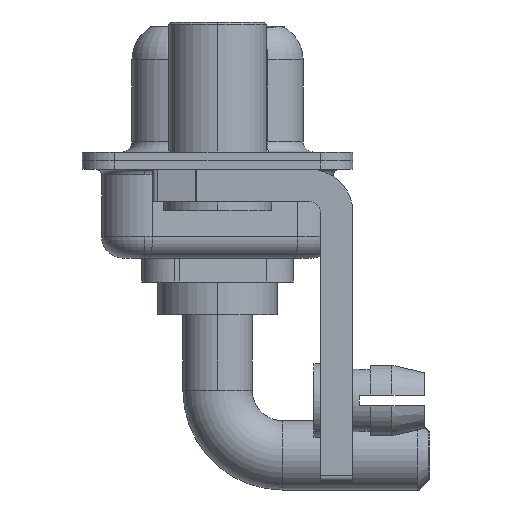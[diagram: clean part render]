
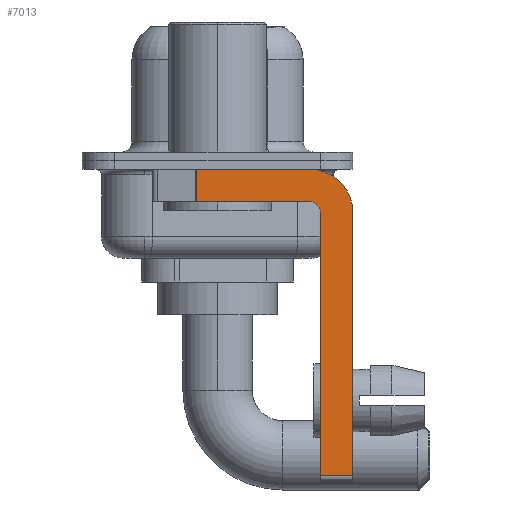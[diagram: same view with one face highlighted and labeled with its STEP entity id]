
A CAD part, left-side view. The second image highlights one B-rep face of the part: STEP entity #7013.
In plain terms, the highlighted planar face has unit normal (-1, 0, 0).
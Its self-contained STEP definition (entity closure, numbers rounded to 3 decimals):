
#165 = AXIS2_PLACEMENT_3D ( 'NONE', #1586, #16486, #4479 ) ;
#211 = CARTESIAN_POINT ( 'NONE',  ( -2.9, -4.25, -2.4 ) ) ;
#673 = LINE ( 'NONE', #15731, #5815 ) ;
#1586 = CARTESIAN_POINT ( 'NONE',  ( -2.9, -4.25, -2.4 ) ) ;
#2033 = CARTESIAN_POINT ( 'NONE',  ( -2.9, -6.25, -2.4 ) ) ;
#2259 = VECTOR ( 'NONE', #5980, 1000. ) ;
#2355 = DIRECTION ( 'NONE',  ( 0., 1., 0. ) ) ;
#2652 = CARTESIAN_POINT ( 'NONE',  ( -2.9, -4.25, -1.9 ) ) ;
#3061 = DIRECTION ( 'NONE',  ( 0., 0., -1. ) ) ;
#3153 = DIRECTION ( 'NONE',  ( 1., 0., 0. ) ) ;
#3361 = LINE ( 'NONE', #2033, #14634 ) ;
#3612 = CARTESIAN_POINT ( 'NONE',  ( -2.9, 0.978, -1.9 ) ) ;
#3843 = ORIENTED_EDGE ( 'NONE', *, *, #8644, .T. ) ;
#4019 = CARTESIAN_POINT ( 'NONE',  ( -2.9, -4.25, -14.55 ) ) ;
#4239 = VECTOR ( 'NONE', #2355, 1000. ) ;
#4290 = CIRCLE ( 'NONE', #7648, 2. ) ;
#4424 = EDGE_CURVE ( 'NONE', #13853, #8016, #9050, .T. ) ;
#4479 = DIRECTION ( 'NONE',  ( 0., 0., 1. ) ) ;
#4519 = AXIS2_PLACEMENT_3D ( 'NONE', #211, #13544, #13622 ) ;
#4754 = ORIENTED_EDGE ( 'NONE', *, *, #17302, .F. ) ;
#4914 = VERTEX_POINT ( 'NONE', #8689 ) ;
#5020 = VECTOR ( 'NONE', #10282, 1000. ) ;
#5219 = ORIENTED_EDGE ( 'NONE', *, *, #14385, .F. ) ;
#5685 = CARTESIAN_POINT ( 'NONE',  ( -2.9, -4.25, -2.4 ) ) ;
#5815 = VECTOR ( 'NONE', #13022, 1000. ) ;
#5980 = DIRECTION ( 'NONE',  ( 0., 0., 1. ) ) ;
#6066 = ORIENTED_EDGE ( 'NONE', *, *, #10455, .F. ) ;
#6239 = CARTESIAN_POINT ( 'NONE',  ( -2.9, -4.75, -14.8 ) ) ;
#6323 = VERTEX_POINT ( 'NONE', #2652 ) ;
#6465 = ORIENTED_EDGE ( 'NONE', *, *, #7728, .F. ) ;
#6474 = LINE ( 'NONE', #15928, #4239 ) ;
#6742 = LINE ( 'NONE', #4019, #8184 ) ;
#7013 = ADVANCED_FACE ( 'NONE', ( #9539 ), #14851, .F. ) ;
#7223 = VERTEX_POINT ( 'NONE', #7839 ) ;
#7386 = DIRECTION ( 'NONE',  ( 0., 0., -1. ) ) ;
#7450 = CIRCLE ( 'NONE', #165, 0.5 ) ;
#7564 = CARTESIAN_POINT ( 'NONE',  ( -2.9, -4.75, -14.55 ) ) ;
#7648 = AXIS2_PLACEMENT_3D ( 'NONE', #5685, #3153, #3061 ) ;
#7728 = EDGE_CURVE ( 'NONE', #11446, #15174, #15430, .T. ) ;
#7839 = CARTESIAN_POINT ( 'NONE',  ( -2.9, -6.25, -14.55 ) ) ;
#8016 = VERTEX_POINT ( 'NONE', #3612 ) ;
#8184 = VECTOR ( 'NONE', #9384, 1000. ) ;
#8410 = EDGE_CURVE ( 'NONE', #6323, #8016, #6474, .T. ) ;
#8644 = EDGE_CURVE ( 'NONE', #11446, #7223, #6742, .T. ) ;
#8689 = CARTESIAN_POINT ( 'NONE',  ( -2.9, -4.25, -0.4 ) ) ;
#8863 = ORIENTED_EDGE ( 'NONE', *, *, #11331, .F. ) ;
#9050 = LINE ( 'NONE', #16914, #5020 ) ;
#9384 = DIRECTION ( 'NONE',  ( 0., -1., 0. ) ) ;
#9539 = FACE_OUTER_BOUND ( 'NONE', #10675, .T. ) ;
#10282 = DIRECTION ( 'NONE',  ( 0., 0., -1. ) ) ;
#10455 = EDGE_CURVE ( 'NONE', #4914, #16020, #4290, .T. ) ;
#10599 = CARTESIAN_POINT ( 'NONE',  ( -2.9, 0.978, -0.4 ) ) ;
#10675 = EDGE_LOOP ( 'NONE', ( #4754, #13245, #10933, #5219, #6465, #3843, #8863, #6066 ) ) ;
#10933 = ORIENTED_EDGE ( 'NONE', *, *, #8410, .F. ) ;
#11331 = EDGE_CURVE ( 'NONE', #16020, #7223, #3361, .T. ) ;
#11446 = VERTEX_POINT ( 'NONE', #7564 ) ;
#12130 = CARTESIAN_POINT ( 'NONE',  ( -2.9, -6.25, -2.4 ) ) ;
#13022 = DIRECTION ( 'NONE',  ( 0., -1., 0. ) ) ;
#13245 = ORIENTED_EDGE ( 'NONE', *, *, #4424, .T. ) ;
#13544 = DIRECTION ( 'NONE',  ( 1., 0., 0. ) ) ;
#13622 = DIRECTION ( 'NONE',  ( 0., 0., -1. ) ) ;
#13853 = VERTEX_POINT ( 'NONE', #10599 ) ;
#14385 = EDGE_CURVE ( 'NONE', #15174, #6323, #7450, .T. ) ;
#14634 = VECTOR ( 'NONE', #7386, 1000. ) ;
#14851 = PLANE ( 'NONE',  #4519 ) ;
#15174 = VERTEX_POINT ( 'NONE', #16519 ) ;
#15430 = LINE ( 'NONE', #6239, #2259 ) ;
#15731 = CARTESIAN_POINT ( 'NONE',  ( -2.9, 3., -0.4 ) ) ;
#15928 = CARTESIAN_POINT ( 'NONE',  ( -2.9, -4.25, -1.9 ) ) ;
#16020 = VERTEX_POINT ( 'NONE', #12130 ) ;
#16486 = DIRECTION ( 'NONE',  ( -1., 0., 0. ) ) ;
#16519 = CARTESIAN_POINT ( 'NONE',  ( -2.9, -4.75, -2.4 ) ) ;
#16914 = CARTESIAN_POINT ( 'NONE',  ( -2.9, 0.978, -1.9 ) ) ;
#17302 = EDGE_CURVE ( 'NONE', #13853, #4914, #673, .T. ) ;
